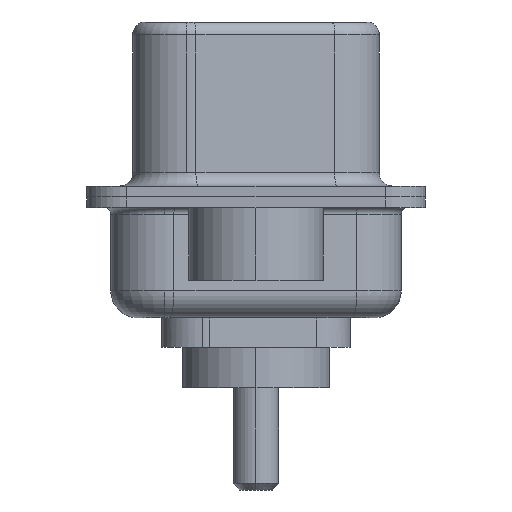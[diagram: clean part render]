
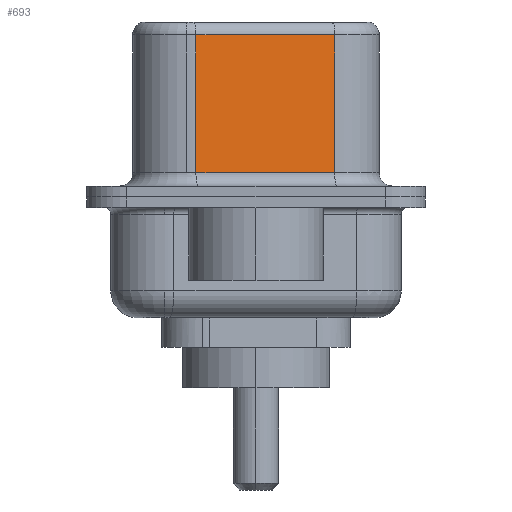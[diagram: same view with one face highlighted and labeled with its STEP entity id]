
A CAD part, left-side view. The second image highlights one B-rep face of the part: STEP entity #693.
In plain terms, the highlighted planar face has unit normal (-0.985, -0.174, 0).
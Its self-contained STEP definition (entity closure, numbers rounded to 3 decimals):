
#219 = ORIENTED_EDGE ( 'NONE', *, *, #5835, .T. ) ;
#693 = ADVANCED_FACE ( 'NONE', ( #13758 ), #9903, .F. ) ;
#748 = ORIENTED_EDGE ( 'NONE', *, *, #1345, .T. ) ;
#1256 = EDGE_CURVE ( 'NONE', #13979, #5256, #11737, .T. ) ;
#1345 = EDGE_CURVE ( 'NONE', #8994, #5256, #8049, .T. ) ;
#2166 = DIRECTION ( 'NONE',  ( 0.985, 0.174, 0. ) ) ;
#2713 = VECTOR ( 'NONE', #12863, 1000. ) ;
#3098 = VERTEX_POINT ( 'NONE', #3286 ) ;
#3286 = CARTESIAN_POINT ( 'NONE',  ( 3.675, 2.233, 6.02 ) ) ;
#4509 = CARTESIAN_POINT ( 'NONE',  ( 3.675, 2.233, 0.9 ) ) ;
#4607 = AXIS2_PLACEMENT_3D ( 'NONE', #5873, #2166, #13359 ) ;
#4629 = LINE ( 'NONE', #5845, #7311 ) ;
#5256 = VERTEX_POINT ( 'NONE', #8512 ) ;
#5690 = VECTOR ( 'NONE', #13032, 1000. ) ;
#5835 = EDGE_CURVE ( 'NONE', #3098, #8994, #14066, .T. ) ;
#5845 = CARTESIAN_POINT ( 'NONE',  ( 4.585, -2.927, 6.02 ) ) ;
#5873 = CARTESIAN_POINT ( 'NONE',  ( 4.585, -2.927, 6.52 ) ) ;
#5931 = DIRECTION ( 'NONE',  ( 0., 0., -1. ) ) ;
#7311 = VECTOR ( 'NONE', #12567, 1000. ) ;
#8049 = LINE ( 'NONE', #13043, #5690 ) ;
#8438 = VECTOR ( 'NONE', #5931, 1000. ) ;
#8512 = CARTESIAN_POINT ( 'NONE',  ( 4.585, -2.927, 0.9 ) ) ;
#8925 = CARTESIAN_POINT ( 'NONE',  ( 4.585, -2.927, 6.02 ) ) ;
#8994 = VERTEX_POINT ( 'NONE', #4509 ) ;
#9867 = CARTESIAN_POINT ( 'NONE',  ( 4.585, -2.927, 6.52 ) ) ;
#9903 = PLANE ( 'NONE',  #4607 ) ;
#9948 = ORIENTED_EDGE ( 'NONE', *, *, #10539, .T. ) ;
#10539 = EDGE_CURVE ( 'NONE', #13979, #3098, #4629, .T. ) ;
#11670 = ORIENTED_EDGE ( 'NONE', *, *, #1256, .F. ) ;
#11737 = LINE ( 'NONE', #9867, #2713 ) ;
#12567 = DIRECTION ( 'NONE',  ( -0.174, 0.985, 0. ) ) ;
#12863 = DIRECTION ( 'NONE',  ( 0., 0., -1. ) ) ;
#12968 = CARTESIAN_POINT ( 'NONE',  ( 3.675, 2.233, 6.52 ) ) ;
#13032 = DIRECTION ( 'NONE',  ( 0.174, -0.985, 0. ) ) ;
#13043 = CARTESIAN_POINT ( 'NONE',  ( 4.585, -2.927, 0.9 ) ) ;
#13230 = EDGE_LOOP ( 'NONE', ( #11670, #9948, #219, #748 ) ) ;
#13359 = DIRECTION ( 'NONE',  ( -0.174, 0.985, 0. ) ) ;
#13758 = FACE_OUTER_BOUND ( 'NONE', #13230, .T. ) ;
#13979 = VERTEX_POINT ( 'NONE', #8925 ) ;
#14066 = LINE ( 'NONE', #12968, #8438 ) ;
